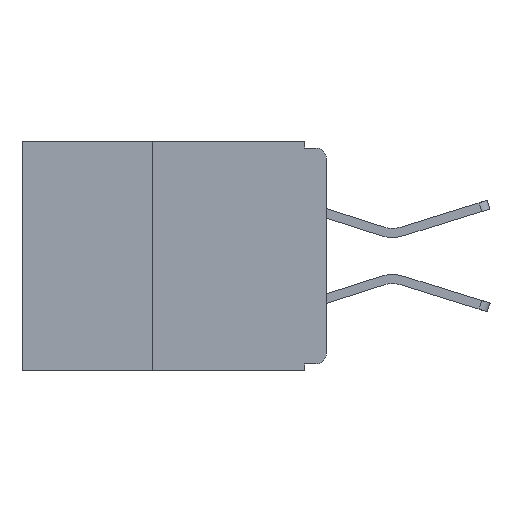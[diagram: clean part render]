
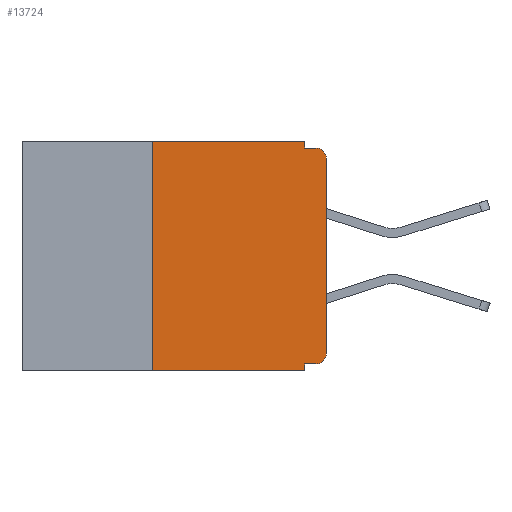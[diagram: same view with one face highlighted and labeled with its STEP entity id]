
A CAD part, left-side view. The second image highlights one B-rep face of the part: STEP entity #13724.
In plain terms, the highlighted planar face has unit normal (-1, 0, 0).
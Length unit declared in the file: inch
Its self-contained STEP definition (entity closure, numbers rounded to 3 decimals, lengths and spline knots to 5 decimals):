
#278 = ORIENTED_EDGE ( 'NONE', *, *, #493, .T. ) ;
#335 = CARTESIAN_POINT ( 'NONE',  ( 0., 0.25, -0.33 ) ) ;
#449 = ORIENTED_EDGE ( 'NONE', *, *, #20781, .T. ) ;
#493 = EDGE_CURVE ( 'NONE', #5932, #9781, #2407, .T. ) ;
#1170 = VERTEX_POINT ( 'NONE', #11902 ) ;
#1501 = ORIENTED_EDGE ( 'NONE', *, *, #6394, .F. ) ;
#1559 = CARTESIAN_POINT ( 'NONE',  ( 0., 0.031, 0. ) ) ;
#1642 = CARTESIAN_POINT ( 'NONE',  ( 0., 0.031, -0.01 ) ) ;
#2373 = ORIENTED_EDGE ( 'NONE', *, *, #5133, .T. ) ;
#2407 = LINE ( 'NONE', #9955, #19540 ) ;
#2950 = EDGE_CURVE ( 'NONE', #1170, #10720, #6682, .T. ) ;
#3097 = EDGE_CURVE ( 'NONE', #9781, #18893, #20714, .T. ) ;
#3139 = CARTESIAN_POINT ( 'NONE',  ( 0., 0.25, 0. ) ) ;
#3446 = LINE ( 'NONE', #17073, #15855 ) ;
#3940 = VERTEX_POINT ( 'NONE', #3139 ) ;
#4009 = VERTEX_POINT ( 'NONE', #1642 ) ;
#4080 = DIRECTION ( 'NONE',  ( 0., 0., -1. ) ) ;
#4202 = CARTESIAN_POINT ( 'NONE',  ( 0., 0.031, -0.33 ) ) ;
#4958 = EDGE_LOOP ( 'NONE', ( #278, #5148, #6718, #8237, #6168, #18112, #2373, #6738, #1501, #449 ) ) ;
#5133 = EDGE_CURVE ( 'NONE', #14432, #10720, #20469, .T. ) ;
#5148 = ORIENTED_EDGE ( 'NONE', *, *, #3097, .T. ) ;
#5241 = CARTESIAN_POINT ( 'NONE',  ( 0., 0.437, 0. ) ) ;
#5400 = CIRCLE ( 'NONE', #10767, 0.015 ) ;
#5593 = LINE ( 'NONE', #15123, #13222 ) ;
#5921 = VECTOR ( 'NONE', #18617, 39.37008 ) ;
#5932 = VERTEX_POINT ( 'NONE', #14566 ) ;
#6044 = CARTESIAN_POINT ( 'NONE',  ( 0., 0.015, -0.32 ) ) ;
#6168 = ORIENTED_EDGE ( 'NONE', *, *, #20735, .F. ) ;
#6394 = EDGE_CURVE ( 'NONE', #19543, #1170, #14956, .T. ) ;
#6682 = LINE ( 'NONE', #4202, #10998 ) ;
#6718 = ORIENTED_EDGE ( 'NONE', *, *, #13991, .F. ) ;
#6738 = ORIENTED_EDGE ( 'NONE', *, *, #2950, .F. ) ;
#6906 = DIRECTION ( 'NONE',  ( 0., 0., -1. ) ) ;
#7096 = DIRECTION ( 'NONE',  ( 0., 0., -1. ) ) ;
#7101 = CARTESIAN_POINT ( 'NONE',  ( 0., 0., -0.025 ) ) ;
#7559 = FACE_OUTER_BOUND ( 'NONE', #4958, .T. ) ;
#8237 = ORIENTED_EDGE ( 'NONE', *, *, #11687, .F. ) ;
#8358 = VERTEX_POINT ( 'NONE', #1559 ) ;
#8437 = EDGE_CURVE ( 'NONE', #14432, #3940, #14398, .T. ) ;
#8904 = DIRECTION ( 'NONE',  ( -1., 0., 0. ) ) ;
#9048 = CARTESIAN_POINT ( 'NONE',  ( 0., 0.437, 0. ) ) ;
#9183 = DIRECTION ( 'NONE',  ( -1., 0., 0. ) ) ;
#9781 = VERTEX_POINT ( 'NONE', #7101 ) ;
#9955 = CARTESIAN_POINT ( 'NONE',  ( 0., 0., 0. ) ) ;
#9983 = DIRECTION ( 'NONE',  ( 0., 0., 1. ) ) ;
#10120 = VECTOR ( 'NONE', #9983, 39.37008 ) ;
#10720 = VERTEX_POINT ( 'NONE', #19031 ) ;
#10767 = AXIS2_PLACEMENT_3D ( 'NONE', #18748, #9183, #20358 ) ;
#10998 = VECTOR ( 'NONE', #4080, 39.37008 ) ;
#11096 = CARTESIAN_POINT ( 'NONE',  ( 0., 0.437, -0.33 ) ) ;
#11687 = EDGE_CURVE ( 'NONE', #8358, #4009, #5593, .T. ) ;
#11718 = PLANE ( 'NONE',  #19623 ) ;
#11902 = CARTESIAN_POINT ( 'NONE',  ( 0., 0.031, -0.32 ) ) ;
#13222 = VECTOR ( 'NONE', #7096, 39.37008 ) ;
#13574 = CARTESIAN_POINT ( 'NONE',  ( 0., 0.015, -0.01 ) ) ;
#13724 = ADVANCED_FACE ( 'NONE', ( #7559 ), #11718, .F. ) ;
#13991 = EDGE_CURVE ( 'NONE', #4009, #18893, #3446, .T. ) ;
#14398 = LINE ( 'NONE', #17885, #10120 ) ;
#14432 = VERTEX_POINT ( 'NONE', #335 ) ;
#14566 = CARTESIAN_POINT ( 'NONE',  ( 0., 0., -0.305 ) ) ;
#14565 = DIRECTION ( 'NONE',  ( 0., 1., 0. ) ) ;
#14956 = LINE ( 'NONE', #20817, #18669 ) ;
#15123 = CARTESIAN_POINT ( 'NONE',  ( 0., 0.031, 0. ) ) ;
#15855 = VECTOR ( 'NONE', #18665, 39.37008 ) ;
#16245 = VECTOR ( 'NONE', #20635, 39.37008 ) ;
#16521 = DIRECTION ( 'NONE',  ( 1., 0., 0. ) ) ;
#17073 = CARTESIAN_POINT ( 'NONE',  ( 0., 0., -0.01 ) ) ;
#17885 = CARTESIAN_POINT ( 'NONE',  ( 0., 0.25, -0.33 ) ) ;
#18112 = ORIENTED_EDGE ( 'NONE', *, *, #8437, .F. ) ;
#18210 = AXIS2_PLACEMENT_3D ( 'NONE', #18475, #8904, #20081 ) ;
#18243 = LINE ( 'NONE', #9048, #5921 ) ;
#18475 = CARTESIAN_POINT ( 'NONE',  ( 0., 0.015, -0.025 ) ) ;
#18617 = DIRECTION ( 'NONE',  ( 0., -1., 0. ) ) ;
#18665 = DIRECTION ( 'NONE',  ( 0., -1., 0. ) ) ;
#18669 = VECTOR ( 'NONE', #14565, 39.37008 ) ;
#18748 = CARTESIAN_POINT ( 'NONE',  ( 0., 0.015, -0.305 ) ) ;
#18848 = DIRECTION ( 'NONE',  ( 0., 0., 1. ) ) ;
#18893 = VERTEX_POINT ( 'NONE', #13574 ) ;
#19031 = CARTESIAN_POINT ( 'NONE',  ( 0., 0.031, -0.33 ) ) ;
#19540 = VECTOR ( 'NONE', #18848, 39.37008 ) ;
#19543 = VERTEX_POINT ( 'NONE', #6044 ) ;
#19623 = AXIS2_PLACEMENT_3D ( 'NONE', #5241, #16521, #6906 ) ;
#20081 = DIRECTION ( 'NONE',  ( 0., 0., -1. ) ) ;
#20358 = DIRECTION ( 'NONE',  ( 0., 0., -1. ) ) ;
#20469 = LINE ( 'NONE', #11096, #16245 ) ;
#20635 = DIRECTION ( 'NONE',  ( 0., -1., 0. ) ) ;
#20714 = CIRCLE ( 'NONE', #18210, 0.015 ) ;
#20735 = EDGE_CURVE ( 'NONE', #3940, #8358, #18243, .T. ) ;
#20781 = EDGE_CURVE ( 'NONE', #19543, #5932, #5400, .T. ) ;
#20817 = CARTESIAN_POINT ( 'NONE',  ( 0., 0., -0.32 ) ) ;
